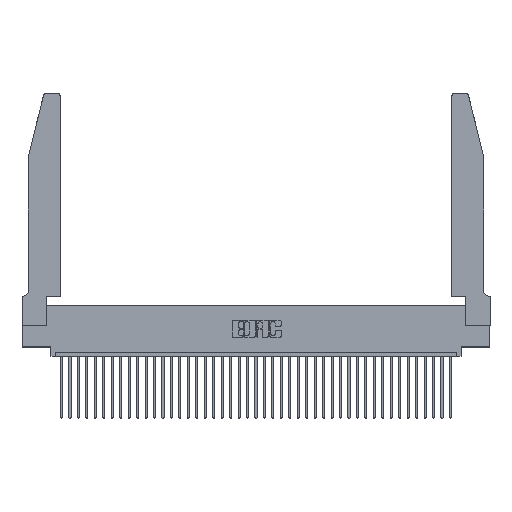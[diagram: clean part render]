
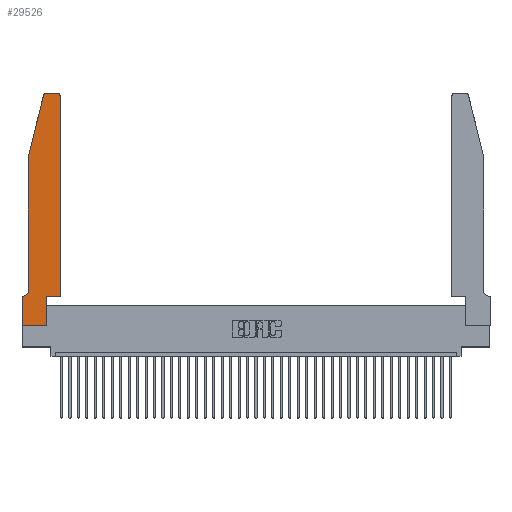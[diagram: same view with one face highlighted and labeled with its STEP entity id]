
A CAD part, top view. The second image highlights one B-rep face of the part: STEP entity #29526.
In plain terms, the highlighted planar face has unit normal (0, 0, 1).
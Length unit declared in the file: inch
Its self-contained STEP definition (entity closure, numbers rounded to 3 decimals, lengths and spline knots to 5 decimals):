
#42 = LINE ( 'NONE', #7655, #468 ) ;
#155 = ORIENTED_EDGE ( 'NONE', *, *, #3860, .T. ) ;
#402 = CARTESIAN_POINT ( 'NONE',  ( 0.2605, 2.75, 0.37 ) ) ;
#468 = VECTOR ( 'NONE', #16634, 39.37008 ) ;
#751 = LINE ( 'NONE', #15178, #2679 ) ;
#1139 = DIRECTION ( 'NONE',  ( 1., 0., 0. ) ) ;
#1884 = CARTESIAN_POINT ( 'NONE',  ( 0.4205, 2.75, 0.37 ) ) ;
#2593 = DIRECTION ( 'NONE',  ( 0., -1., 0. ) ) ;
#2679 = VECTOR ( 'NONE', #12236, 39.37008 ) ;
#2854 = VERTEX_POINT ( 'NONE', #37560 ) ;
#3403 = EDGE_CURVE ( 'NONE', #2854, #19723, #35677, .T. ) ;
#3860 = EDGE_CURVE ( 'NONE', #3985, #36988, #751, .T. ) ;
#3985 = VERTEX_POINT ( 'NONE', #4148 ) ;
#4148 = CARTESIAN_POINT ( 'NONE',  ( 0.2865, 0., 0.37 ) ) ;
#4510 = CARTESIAN_POINT ( 'NONE',  ( 0., 0., 0.37 ) ) ;
#5056 = VECTOR ( 'NONE', #20713, 39.37008 ) ;
#5420 = CARTESIAN_POINT ( 'NONE',  ( 0.0755, 0.35, 0.37 ) ) ;
#6027 = LINE ( 'NONE', #17930, #5056 ) ;
#6242 = VERTEX_POINT ( 'NONE', #15128 ) ;
#7595 = DIRECTION ( 'NONE',  ( 1., 0., 0. ) ) ;
#7655 = CARTESIAN_POINT ( 'NONE',  ( 0.4505, 0.35, 0.37 ) ) ;
#8812 = CARTESIAN_POINT ( 'NONE',  ( 0.0055, 0.42, 0.37 ) ) ;
#9004 = DIRECTION ( 'NONE',  ( 1., 0., 0. ) ) ;
#9636 = DIRECTION ( 'NONE',  ( 0., 0., 1. ) ) ;
#9717 = LINE ( 'NONE', #24958, #39366 ) ;
#9901 = DIRECTION ( 'NONE',  ( 1., 0., 0. ) ) ;
#10129 = VERTEX_POINT ( 'NONE', #37595 ) ;
#10291 = FACE_OUTER_BOUND ( 'NONE', #17287, .T. ) ;
#10594 = CARTESIAN_POINT ( 'NONE',  ( 0., 0., 0.37 ) ) ;
#11563 = CARTESIAN_POINT ( 'NONE',  ( 0.0755, 2., 0.37 ) ) ;
#12070 = VECTOR ( 'NONE', #2593, 39.37008 ) ;
#12236 = DIRECTION ( 'NONE',  ( 0., 1., 0. ) ) ;
#13092 = EDGE_CURVE ( 'NONE', #18195, #3985, #34682, .T. ) ;
#14537 = ORIENTED_EDGE ( 'NONE', *, *, #31474, .T. ) ;
#15128 = CARTESIAN_POINT ( 'NONE',  ( 0.0755, 2., 0.37 ) ) ;
#15178 = CARTESIAN_POINT ( 'NONE',  ( 0.2865, 0.35, 0.37 ) ) ;
#16173 = CARTESIAN_POINT ( 'NONE',  ( 0.25487, 2.72718, 0.37 ) ) ;
#16634 = DIRECTION ( 'NONE',  ( 0., 1., 0. ) ) ;
#16857 = CARTESIAN_POINT ( 'NONE',  ( 0.284, 2.75, 0.37 ) ) ;
#17046 = VECTOR ( 'NONE', #1139, 39.37008 ) ;
#17287 = EDGE_LOOP ( 'NONE', ( #34723, #17976, #14537, #35272, #29847, #18908, #26672, #30143, #155, #23881, #39475, #18367 ) ) ;
#17801 = DIRECTION ( 'NONE',  ( -1., 0., 0. ) ) ;
#17930 = CARTESIAN_POINT ( 'NONE',  ( 0.4505, 0.35, 0.37 ) ) ;
#17976 = ORIENTED_EDGE ( 'NONE', *, *, #25314, .T. ) ;
#18195 = VERTEX_POINT ( 'NONE', #10594 ) ;
#18367 = ORIENTED_EDGE ( 'NONE', *, *, #29178, .T. ) ;
#18401 = VERTEX_POINT ( 'NONE', #1884 ) ;
#18625 = LINE ( 'NONE', #11563, #25749 ) ;
#18908 = ORIENTED_EDGE ( 'NONE', *, *, #20648, .T. ) ;
#19532 = CARTESIAN_POINT ( 'NONE',  ( 0., 0.35, 0.37 ) ) ;
#19723 = VERTEX_POINT ( 'NONE', #20341 ) ;
#20157 = CIRCLE ( 'NONE', #21254, 0.03 ) ;
#20341 = CARTESIAN_POINT ( 'NONE',  ( 0.0055, 0.35, 0.37 ) ) ;
#20648 = EDGE_CURVE ( 'NONE', #19723, #10129, #31713, .T. ) ;
#20713 = DIRECTION ( 'NONE',  ( 1., 0., 0. ) ) ;
#21165 = CARTESIAN_POINT ( 'NONE',  ( 0.4505, 2.72, 0.37 ) ) ;
#21254 = AXIS2_PLACEMENT_3D ( 'NONE', #26940, #36114, #9004 ) ;
#21939 = CARTESIAN_POINT ( 'NONE',  ( 0.4205, 2.72, 0.37 ) ) ;
#23872 = AXIS2_PLACEMENT_3D ( 'NONE', #21939, #9636, #9901 ) ;
#23881 = ORIENTED_EDGE ( 'NONE', *, *, #29721, .T. ) ;
#23902 = EDGE_CURVE ( 'NONE', #18401, #25061, #34114, .T. ) ;
#24088 = DIRECTION ( 'NONE',  ( -1., 0., 0. ) ) ;
#24958 = CARTESIAN_POINT ( 'NONE',  ( 0.0755, 2., 0.37 ) ) ;
#25061 = VERTEX_POINT ( 'NONE', #16857 ) ;
#25314 = EDGE_CURVE ( 'NONE', #25061, #31064, #20157, .T. ) ;
#25522 = VECTOR ( 'NONE', #24088, 39.37008 ) ;
#25749 = VECTOR ( 'NONE', #35989, 39.37008 ) ;
#25765 = CARTESIAN_POINT ( 'NONE',  ( 0.4505, 0.35, 0.37 ) ) ;
#26672 = ORIENTED_EDGE ( 'NONE', *, *, #31888, .T. ) ;
#26939 = CARTESIAN_POINT ( 'NONE',  ( 0., 0., 0.37 ) ) ;
#26940 = CARTESIAN_POINT ( 'NONE',  ( 0.284, 2.72, 0.37 ) ) ;
#27571 = CIRCLE ( 'NONE', #23872, 0.03 ) ;
#28070 = DIRECTION ( 'NONE',  ( -1., 0., 0. ) ) ;
#29080 = VERTEX_POINT ( 'NONE', #21165 ) ;
#29178 = EDGE_CURVE ( 'NONE', #29080, #18401, #27571, .T. ) ;
#29526 = ADVANCED_FACE ( 'NONE', ( #10291 ), #31633, .T. ) ;
#29721 = EDGE_CURVE ( 'NONE', #36988, #36791, #6027, .T. ) ;
#29847 = ORIENTED_EDGE ( 'NONE', *, *, #3403, .T. ) ;
#30047 = CARTESIAN_POINT ( 'NONE',  ( 0.2865, 0.35, 0.37 ) ) ;
#30143 = ORIENTED_EDGE ( 'NONE', *, *, #13092, .T. ) ;
#30339 = DIRECTION ( 'NONE',  ( 0., 0., -1. ) ) ;
#31064 = VERTEX_POINT ( 'NONE', #16173 ) ;
#31474 = EDGE_CURVE ( 'NONE', #31064, #6242, #9717, .T. ) ;
#31633 = PLANE ( 'NONE',  #35142 ) ;
#31713 = LINE ( 'NONE', #5420, #25522 ) ;
#31888 = EDGE_CURVE ( 'NONE', #10129, #18195, #38354, .T. ) ;
#32185 = VECTOR ( 'NONE', #28070, 39.37008 ) ;
#34114 = LINE ( 'NONE', #402, #32185 ) ;
#34242 = EDGE_CURVE ( 'NONE', #6242, #2854, #18625, .T. ) ;
#34682 = LINE ( 'NONE', #4510, #17046 ) ;
#34723 = ORIENTED_EDGE ( 'NONE', *, *, #23902, .T. ) ;
#35121 = DIRECTION ( 'NONE',  ( 0., 0., 1. ) ) ;
#35142 = AXIS2_PLACEMENT_3D ( 'NONE', #19532, #35121, #7595 ) ;
#35272 = ORIENTED_EDGE ( 'NONE', *, *, #34242, .T. ) ;
#35677 = CIRCLE ( 'NONE', #37888, 0.07 ) ;
#35989 = DIRECTION ( 'NONE',  ( 0., -1., 0. ) ) ;
#36114 = DIRECTION ( 'NONE',  ( 0., 0., 1. ) ) ;
#36532 = EDGE_CURVE ( 'NONE', #36791, #29080, #42, .T. ) ;
#36791 = VERTEX_POINT ( 'NONE', #25765 ) ;
#36988 = VERTEX_POINT ( 'NONE', #30047 ) ;
#37077 = DIRECTION ( 'NONE',  ( -0.239, -0.971, 0. ) ) ;
#37560 = CARTESIAN_POINT ( 'NONE',  ( 0.0755, 0.42, 0.37 ) ) ;
#37595 = CARTESIAN_POINT ( 'NONE',  ( 0., 0.35, 0.37 ) ) ;
#37888 = AXIS2_PLACEMENT_3D ( 'NONE', #8812, #30339, #17801 ) ;
#38354 = LINE ( 'NONE', #26939, #12070 ) ;
#39366 = VECTOR ( 'NONE', #37077, 39.37008 ) ;
#39475 = ORIENTED_EDGE ( 'NONE', *, *, #36532, .T. ) ;
